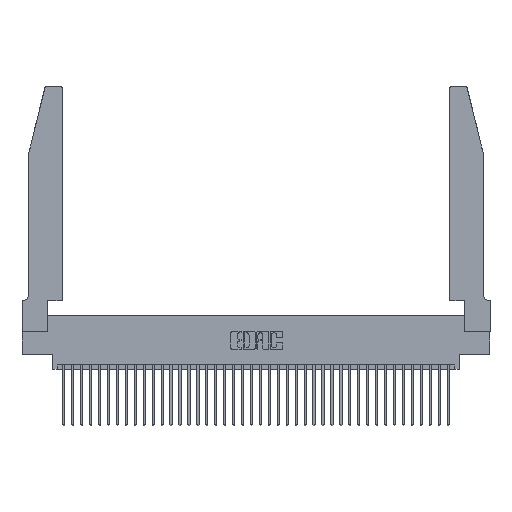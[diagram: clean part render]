
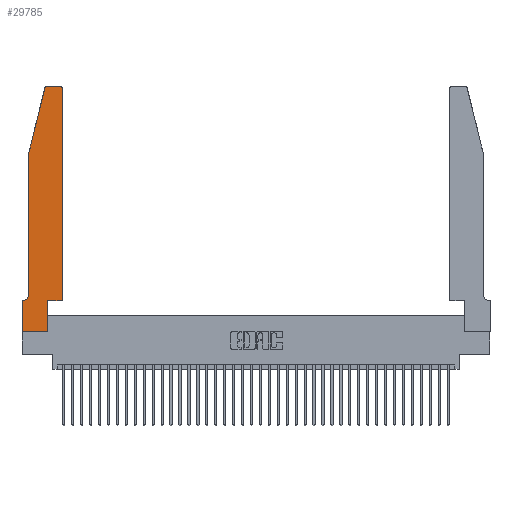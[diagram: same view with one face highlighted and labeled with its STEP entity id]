
A CAD part, top view. The second image highlights one B-rep face of the part: STEP entity #29785.
In plain terms, the highlighted planar face has unit normal (0, 0, 1).
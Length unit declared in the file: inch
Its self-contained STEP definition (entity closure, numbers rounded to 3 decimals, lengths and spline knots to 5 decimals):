
#38 = VERTEX_POINT ( 'NONE', #12372 ) ;
#706 = PLANE ( 'NONE',  #30173 ) ;
#1243 = CARTESIAN_POINT ( 'NONE',  ( 0.0055, 0.42, 0.37 ) ) ;
#2017 = VERTEX_POINT ( 'NONE', #5237 ) ;
#2099 = DIRECTION ( 'NONE',  ( -1., 0., 0. ) ) ;
#2470 = VECTOR ( 'NONE', #37244, 39.37008 ) ;
#3006 = CARTESIAN_POINT ( 'NONE',  ( 0., 0., 0.37 ) ) ;
#3750 = AXIS2_PLACEMENT_3D ( 'NONE', #23816, #5602, #26804 ) ;
#3804 = CARTESIAN_POINT ( 'NONE',  ( 0.4505, 0.35, 0.37 ) ) ;
#3859 = DIRECTION ( 'NONE',  ( 1., 0., 0. ) ) ;
#3988 = CARTESIAN_POINT ( 'NONE',  ( 0.0755, 0.42, 0.37 ) ) ;
#4221 = LINE ( 'NONE', #31511, #27466 ) ;
#4256 = CARTESIAN_POINT ( 'NONE',  ( 0.284, 2.72, 0.37 ) ) ;
#4372 = DIRECTION ( 'NONE',  ( -1., 0., 0. ) ) ;
#4580 = ORIENTED_EDGE ( 'NONE', *, *, #14697, .T. ) ;
#4657 = CIRCLE ( 'NONE', #28541, 0.07 ) ;
#4663 = ORIENTED_EDGE ( 'NONE', *, *, #19110, .T. ) ;
#4672 = CARTESIAN_POINT ( 'NONE',  ( 0., 0.35, 0.37 ) ) ;
#5237 = CARTESIAN_POINT ( 'NONE',  ( 0.4505, 0.35, 0.37 ) ) ;
#5313 = CARTESIAN_POINT ( 'NONE',  ( 0.25487, 2.72718, 0.37 ) ) ;
#5510 = EDGE_CURVE ( 'NONE', #12238, #24518, #29722, .T. ) ;
#5590 = CIRCLE ( 'NONE', #3750, 0.03 ) ;
#5602 = DIRECTION ( 'NONE',  ( 0., 0., 1. ) ) ;
#5805 = VERTEX_POINT ( 'NONE', #5929 ) ;
#5929 = CARTESIAN_POINT ( 'NONE',  ( 0.0055, 0.35, 0.37 ) ) ;
#6764 = CARTESIAN_POINT ( 'NONE',  ( 0.4505, 0.35, 0.37 ) ) ;
#7325 = DIRECTION ( 'NONE',  ( 1., 0., 0. ) ) ;
#7496 = VECTOR ( 'NONE', #37679, 39.37008 ) ;
#7498 = DIRECTION ( 'NONE',  ( -1., 0., 0. ) ) ;
#7633 = CARTESIAN_POINT ( 'NONE',  ( 0.2865, 0.35, 0.37 ) ) ;
#9860 = AXIS2_PLACEMENT_3D ( 'NONE', #4256, #25506, #7325 ) ;
#10424 = CARTESIAN_POINT ( 'NONE',  ( 0.0755, 2., 0.37 ) ) ;
#11065 = VERTEX_POINT ( 'NONE', #4672 ) ;
#11609 = DIRECTION ( 'NONE',  ( 1., 0., 0. ) ) ;
#11651 = CARTESIAN_POINT ( 'NONE',  ( 0.2865, 0., 0.37 ) ) ;
#12238 = VERTEX_POINT ( 'NONE', #11651 ) ;
#12372 = CARTESIAN_POINT ( 'NONE',  ( 0.4205, 2.75, 0.37 ) ) ;
#12633 = EDGE_CURVE ( 'NONE', #20770, #17449, #27189, .T. ) ;
#14677 = CARTESIAN_POINT ( 'NONE',  ( 0., 0., 0.37 ) ) ;
#14697 = EDGE_CURVE ( 'NONE', #5805, #11065, #38023, .T. ) ;
#14772 = EDGE_CURVE ( 'NONE', #14906, #12238, #20248, .T. ) ;
#14906 = VERTEX_POINT ( 'NONE', #15333 ) ;
#15028 = VECTOR ( 'NONE', #2099, 39.37008 ) ;
#15043 = VERTEX_POINT ( 'NONE', #25105 ) ;
#15333 = CARTESIAN_POINT ( 'NONE',  ( 0., 0., 0.37 ) ) ;
#15613 = EDGE_CURVE ( 'NONE', #2017, #15043, #30933, .T. ) ;
#16004 = CARTESIAN_POINT ( 'NONE',  ( 0., 0.35, 0.37 ) ) ;
#16076 = DIRECTION ( 'NONE',  ( 1., 0., 0. ) ) ;
#16894 = EDGE_LOOP ( 'NONE', ( #17344, #20160, #21105, #25569, #36623, #4580, #4663, #25902, #22047, #17239, #30222, #34168 ) ) ;
#17239 = ORIENTED_EDGE ( 'NONE', *, *, #35009, .T. ) ;
#17344 = ORIENTED_EDGE ( 'NONE', *, *, #24502, .T. ) ;
#17449 = VERTEX_POINT ( 'NONE', #36282 ) ;
#18921 = VECTOR ( 'NONE', #16076, 39.37008 ) ;
#19110 = EDGE_CURVE ( 'NONE', #11065, #14906, #29804, .T. ) ;
#19194 = CIRCLE ( 'NONE', #9860, 0.03 ) ;
#19661 = LINE ( 'NONE', #31241, #2470 ) ;
#19921 = CARTESIAN_POINT ( 'NONE',  ( 0.284, 2.75, 0.37 ) ) ;
#20138 = VECTOR ( 'NONE', #22527, 39.37008 ) ;
#20160 = ORIENTED_EDGE ( 'NONE', *, *, #22488, .T. ) ;
#20248 = LINE ( 'NONE', #14677, #27301 ) ;
#20770 = VERTEX_POINT ( 'NONE', #5313 ) ;
#21105 = ORIENTED_EDGE ( 'NONE', *, *, #12633, .T. ) ;
#21252 = DIRECTION ( 'NONE',  ( 0., -1., 0. ) ) ;
#21852 = VECTOR ( 'NONE', #21252, 39.37008 ) ;
#22047 = ORIENTED_EDGE ( 'NONE', *, *, #5510, .T. ) ;
#22069 = VECTOR ( 'NONE', #27931, 39.37008 ) ;
#22077 = DIRECTION ( 'NONE',  ( 0., 0., 1. ) ) ;
#22488 = EDGE_CURVE ( 'NONE', #23085, #20770, #19194, .T. ) ;
#22527 = DIRECTION ( 'NONE',  ( -0.239, -0.971, 0. ) ) ;
#22613 = DIRECTION ( 'NONE',  ( 0., 0., -1. ) ) ;
#23085 = VERTEX_POINT ( 'NONE', #19921 ) ;
#23440 = CARTESIAN_POINT ( 'NONE',  ( 0.0755, 0.35, 0.37 ) ) ;
#23816 = CARTESIAN_POINT ( 'NONE',  ( 0.4205, 2.72, 0.37 ) ) ;
#24502 = EDGE_CURVE ( 'NONE', #38, #23085, #4221, .T. ) ;
#24518 = VERTEX_POINT ( 'NONE', #7633 ) ;
#25105 = CARTESIAN_POINT ( 'NONE',  ( 0.4505, 2.72, 0.37 ) ) ;
#25506 = DIRECTION ( 'NONE',  ( 0., 0., 1. ) ) ;
#25569 = ORIENTED_EDGE ( 'NONE', *, *, #31042, .T. ) ;
#25902 = ORIENTED_EDGE ( 'NONE', *, *, #14772, .T. ) ;
#26804 = DIRECTION ( 'NONE',  ( 1., 0., 0. ) ) ;
#26905 = LINE ( 'NONE', #3804, #18921 ) ;
#27189 = LINE ( 'NONE', #10424, #20138 ) ;
#27301 = VECTOR ( 'NONE', #11609, 39.37008 ) ;
#27466 = VECTOR ( 'NONE', #7498, 39.37008 ) ;
#27563 = EDGE_CURVE ( 'NONE', #15043, #38, #5590, .T. ) ;
#27931 = DIRECTION ( 'NONE',  ( 0., 1., 0. ) ) ;
#28541 = AXIS2_PLACEMENT_3D ( 'NONE', #1243, #22613, #4372 ) ;
#28839 = CARTESIAN_POINT ( 'NONE',  ( 0.2865, 0.35, 0.37 ) ) ;
#29722 = LINE ( 'NONE', #28839, #7496 ) ;
#29785 = ADVANCED_FACE ( 'NONE', ( #32873 ), #706, .T. ) ;
#29804 = LINE ( 'NONE', #3006, #21852 ) ;
#30173 = AXIS2_PLACEMENT_3D ( 'NONE', #16004, #22077, #3859 ) ;
#30222 = ORIENTED_EDGE ( 'NONE', *, *, #15613, .T. ) ;
#30933 = LINE ( 'NONE', #6764, #22069 ) ;
#31042 = EDGE_CURVE ( 'NONE', #17449, #37588, #19661, .T. ) ;
#31241 = CARTESIAN_POINT ( 'NONE',  ( 0.0755, 2., 0.37 ) ) ;
#31511 = CARTESIAN_POINT ( 'NONE',  ( 0.2605, 2.75, 0.37 ) ) ;
#32873 = FACE_OUTER_BOUND ( 'NONE', #16894, .T. ) ;
#34168 = ORIENTED_EDGE ( 'NONE', *, *, #27563, .T. ) ;
#34533 = EDGE_CURVE ( 'NONE', #37588, #5805, #4657, .T. ) ;
#35009 = EDGE_CURVE ( 'NONE', #24518, #2017, #26905, .T. ) ;
#36282 = CARTESIAN_POINT ( 'NONE',  ( 0.0755, 2., 0.37 ) ) ;
#36623 = ORIENTED_EDGE ( 'NONE', *, *, #34533, .T. ) ;
#37244 = DIRECTION ( 'NONE',  ( 0., -1., 0. ) ) ;
#37588 = VERTEX_POINT ( 'NONE', #3988 ) ;
#37679 = DIRECTION ( 'NONE',  ( 0., 1., 0. ) ) ;
#38023 = LINE ( 'NONE', #23440, #15028 ) ;
